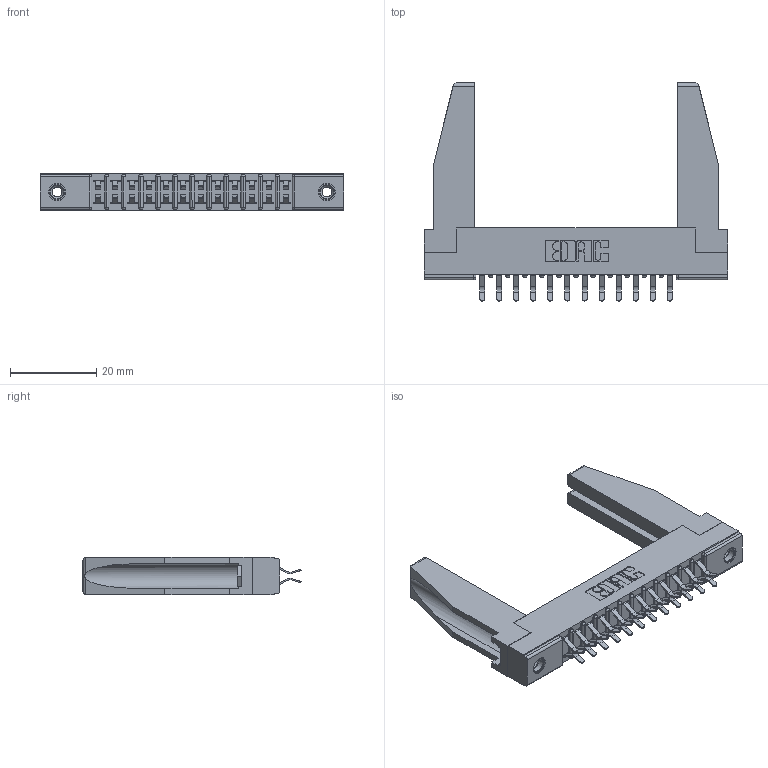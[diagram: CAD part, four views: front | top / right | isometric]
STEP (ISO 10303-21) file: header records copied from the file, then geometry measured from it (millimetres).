
FILE_DESCRIPTION (( 'STEP AP203' ), '1' );
FILE_NAME ('357-024-556-278.STEP', '2019-09-17T22:17:19', ( '' ), ( '' ), 'SwSTEP 2.0', 'SolidWorks 2016', '' );
FILE_SCHEMA (( 'CONFIG_CONTROL_DESIGN' ));
Length unit declared in the file: inch
Products named in the file (5): 307-290-001_556; 307-220-078; 357-024-556-278; 307 Part_.156 Dia Mounting Holes; 345-250-001_345-250-001-102
Assembly tree (29 placements, depth 2):
  357-024-556-278
    307 Part_.156 Dia Mounting Holes
    307-290-001_556  x24
    307-220-078  x2
    345-250-001_345-250-001-102  x2
Bounding box: 70.56 x 50.67 x 8.71 mm (x, y, z)
Volume: 8605.6 mm3; surface area: 11424.9 mm2
Topology: 29 solids, 29 shells, 1461 faces, 4061 edges, 2630 vertices
Faces by surface type: plane 946, cylinder 473, sphere 26, cone 12, torus 4
Entity records: 16913 total; most frequent: CARTESIAN_POINT 2786, ORIENTED_EDGE 2716, DIRECTION 2696, EDGE_CURVE 1358, VECTOR 1032, LINE 1032, VERTEX_POINT 880, AXIS2_PLACEMENT_3D 832
